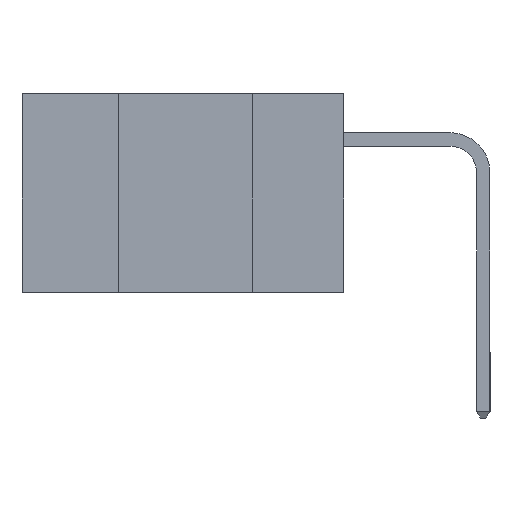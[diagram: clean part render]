
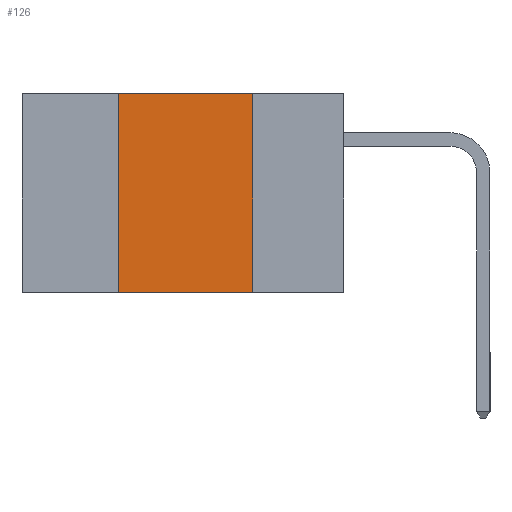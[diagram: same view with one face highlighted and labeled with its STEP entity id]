
A CAD part, left-side view. The second image highlights one B-rep face of the part: STEP entity #126.
In plain terms, the highlighted planar face has unit normal (-1, 0, 0).
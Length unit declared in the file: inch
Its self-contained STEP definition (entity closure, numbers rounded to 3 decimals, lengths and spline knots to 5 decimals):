
#126 = ADVANCED_FACE ( 'NONE', ( #5804 ), #9662, .F. ) ;
#156 = CARTESIAN_POINT ( 'NONE',  ( 0., 0.17, -0.37 ) ) ;
#899 = DIRECTION ( 'NONE',  ( 0., -1., 0. ) ) ;
#2070 = CARTESIAN_POINT ( 'NONE',  ( 0., 0.6, 0. ) ) ;
#2293 = CARTESIAN_POINT ( 'NONE',  ( 0., 0.6, -0.37 ) ) ;
#3684 = VECTOR ( 'NONE', #5436, 39.37008 ) ;
#4465 = AXIS2_PLACEMENT_3D ( 'NONE', #2070, #7155, #6981 ) ;
#4621 = LINE ( 'NONE', #2293, #11092 ) ;
#4655 = DIRECTION ( 'NONE',  ( 0., -1., 0. ) ) ;
#4751 = CARTESIAN_POINT ( 'NONE',  ( 0., 0.17, -0.37 ) ) ;
#5400 = ORIENTED_EDGE ( 'NONE', *, *, #9385, .F. ) ;
#5436 = DIRECTION ( 'NONE',  ( 0., 0., 1. ) ) ;
#5804 = FACE_OUTER_BOUND ( 'NONE', #15985, .T. ) ;
#5898 = CARTESIAN_POINT ( 'NONE',  ( 0., 0.6, 0. ) ) ;
#6466 = LINE ( 'NONE', #156, #13118 ) ;
#6981 = DIRECTION ( 'NONE',  ( 0., 0., -1. ) ) ;
#7155 = DIRECTION ( 'NONE',  ( 1., 0., 0. ) ) ;
#7167 = LINE ( 'NONE', #5898, #15378 ) ;
#8894 = VERTEX_POINT ( 'NONE', #4751 ) ;
#9385 = EDGE_CURVE ( 'NONE', #12977, #15471, #7167, .T. ) ;
#9662 = PLANE ( 'NONE',  #4465 ) ;
#10991 = CARTESIAN_POINT ( 'NONE',  ( 0., 0.42, 0. ) ) ;
#11092 = VECTOR ( 'NONE', #899, 39.37008 ) ;
#11502 = CARTESIAN_POINT ( 'NONE',  ( 0., 0.42, -0.37 ) ) ;
#11667 = DIRECTION ( 'NONE',  ( 0., 0., -1. ) ) ;
#11808 = CARTESIAN_POINT ( 'NONE',  ( 0., 0.42, -0.37 ) ) ;
#12053 = ORIENTED_EDGE ( 'NONE', *, *, #14800, .F. ) ;
#12200 = EDGE_CURVE ( 'NONE', #15471, #8894, #6466, .T. ) ;
#12977 = VERTEX_POINT ( 'NONE', #10991 ) ;
#13118 = VECTOR ( 'NONE', #11667, 39.37008 ) ;
#13300 = VERTEX_POINT ( 'NONE', #11502 ) ;
#13506 = EDGE_CURVE ( 'NONE', #13300, #8894, #4621, .T. ) ;
#14666 = ORIENTED_EDGE ( 'NONE', *, *, #12200, .F. ) ;
#14800 = EDGE_CURVE ( 'NONE', #13300, #12977, #15632, .T. ) ;
#14942 = CARTESIAN_POINT ( 'NONE',  ( 0., 0.17, 0. ) ) ;
#15378 = VECTOR ( 'NONE', #4655, 39.37008 ) ;
#15471 = VERTEX_POINT ( 'NONE', #14942 ) ;
#15632 = LINE ( 'NONE', #11808, #3684 ) ;
#15697 = ORIENTED_EDGE ( 'NONE', *, *, #13506, .T. ) ;
#15985 = EDGE_LOOP ( 'NONE', ( #14666, #5400, #12053, #15697 ) ) ;
